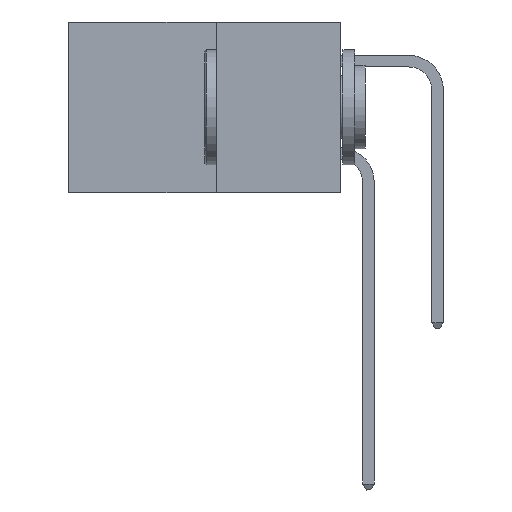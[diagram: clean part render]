
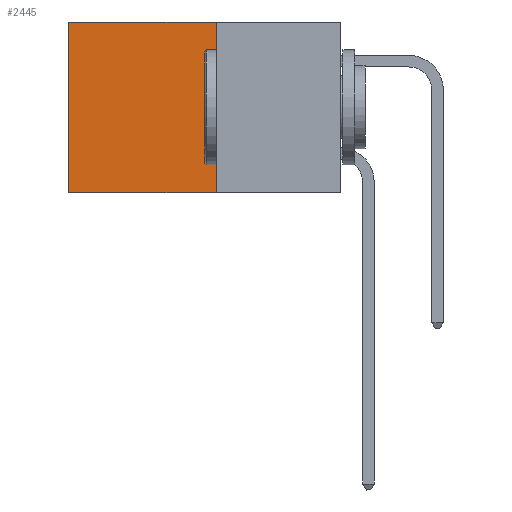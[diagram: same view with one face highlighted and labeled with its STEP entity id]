
A CAD part, left-side view. The second image highlights one B-rep face of the part: STEP entity #2445.
In plain terms, the highlighted planar face has unit normal (-1, 0, 0).
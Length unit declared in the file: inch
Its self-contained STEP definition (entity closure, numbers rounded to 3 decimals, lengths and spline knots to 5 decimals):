
#761 = VERTEX_POINT ( 'NONE', #4590 ) ;
#1286 = LINE ( 'NONE', #3341, #9721 ) ;
#1494 = EDGE_CURVE ( 'NONE', #5302, #4903, #5620, .T. ) ;
#1739 = LINE ( 'NONE', #6395, #7991 ) ;
#2079 = DIRECTION ( 'NONE',  ( 0., 0., -1. ) ) ;
#2236 = VERTEX_POINT ( 'NONE', #6563 ) ;
#2445 = ADVANCED_FACE ( 'NONE', ( #7113 ), #3446, .F. ) ;
#2893 = EDGE_CURVE ( 'NONE', #2236, #761, #1286, .T. ) ;
#3256 = DIRECTION ( 'NONE',  ( 0., 0., -1. ) ) ;
#3278 = DIRECTION ( 'NONE',  ( 1., 0., 0. ) ) ;
#3341 = CARTESIAN_POINT ( 'NONE',  ( 0.277, 0.27, -0.37 ) ) ;
#3374 = CARTESIAN_POINT ( 'NONE',  ( 0.277, 0.27, -0.37 ) ) ;
#3446 = PLANE ( 'NONE',  #8604 ) ;
#3831 = ORIENTED_EDGE ( 'NONE', *, *, #2893, .F. ) ;
#4111 = CARTESIAN_POINT ( 'NONE',  ( 0.277, 0.59, -0.37 ) ) ;
#4160 = DIRECTION ( 'NONE',  ( 0., 1., 0. ) ) ;
#4590 = CARTESIAN_POINT ( 'NONE',  ( 0.277, 0.27, -0.37 ) ) ;
#4757 = DIRECTION ( 'NONE',  ( 0., 0., -1. ) ) ;
#4903 = VERTEX_POINT ( 'NONE', #4111 ) ;
#5302 = VERTEX_POINT ( 'NONE', #7446 ) ;
#5620 = LINE ( 'NONE', #6682, #7761 ) ;
#5762 = ORIENTED_EDGE ( 'NONE', *, *, #1494, .T. ) ;
#6010 = ORIENTED_EDGE ( 'NONE', *, *, #8841, .T. ) ;
#6387 = DIRECTION ( 'NONE',  ( 0., 1., 0. ) ) ;
#6395 = CARTESIAN_POINT ( 'NONE',  ( 0.277, 0.27, -0.37 ) ) ;
#6563 = CARTESIAN_POINT ( 'NONE',  ( 0.277, 0.27, 0. ) ) ;
#6570 = VECTOR ( 'NONE', #4160, 39.37008 ) ;
#6682 = CARTESIAN_POINT ( 'NONE',  ( 0.277, 0.59, -0.37 ) ) ;
#6981 = EDGE_CURVE ( 'NONE', #761, #4903, #1739, .T. ) ;
#7113 = FACE_OUTER_BOUND ( 'NONE', #9545, .T. ) ;
#7446 = CARTESIAN_POINT ( 'NONE',  ( 0.277, 0.59, 0. ) ) ;
#7761 = VECTOR ( 'NONE', #4757, 39.37008 ) ;
#7905 = ORIENTED_EDGE ( 'NONE', *, *, #6981, .F. ) ;
#7991 = VECTOR ( 'NONE', #6387, 39.37008 ) ;
#8206 = CARTESIAN_POINT ( 'NONE',  ( 0.277, 0.27, 0. ) ) ;
#8604 = AXIS2_PLACEMENT_3D ( 'NONE', #3374, #3278, #3256 ) ;
#8713 = LINE ( 'NONE', #8206, #6570 ) ;
#8841 = EDGE_CURVE ( 'NONE', #2236, #5302, #8713, .T. ) ;
#9545 = EDGE_LOOP ( 'NONE', ( #5762, #7905, #3831, #6010 ) ) ;
#9721 = VECTOR ( 'NONE', #2079, 39.37008 ) ;
